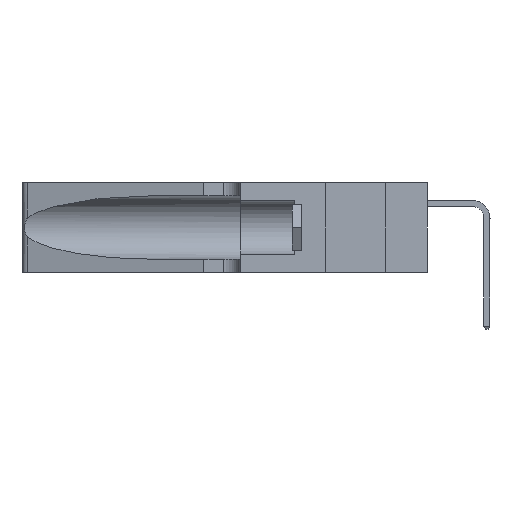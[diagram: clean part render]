
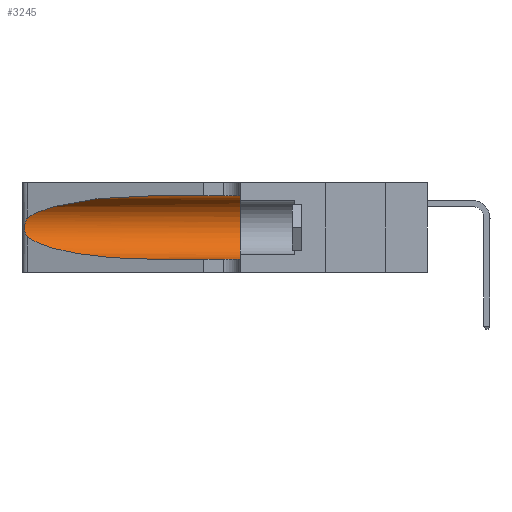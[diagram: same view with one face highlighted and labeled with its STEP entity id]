
A CAD part, left-side view. The second image highlights one B-rep face of the part: STEP entity #3245.
In plain terms, the highlighted cylindrical face has radius 3.308 mm (diameter 6.617 mm), a partial arc.
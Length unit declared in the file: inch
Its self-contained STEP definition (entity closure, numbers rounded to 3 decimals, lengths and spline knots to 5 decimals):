
#115 = EDGE_LOOP ( 'NONE', ( #27801, #45926, #17622, #12856, #36466, #26575 ) ) ;
#1386 = EDGE_CURVE ( 'NONE', #31022, #13780, #26283, .T. ) ;
#2313 = CARTESIAN_POINT ( 'NONE',  ( 0.2373, 1.15595, 0.08982 ) ) ;
#2814 = CARTESIAN_POINT ( 'NONE',  ( 0.26075, 1.23896, 0.19203 ) ) ;
#3019 = CARTESIAN_POINT ( 'NONE',  ( 0.1305, 0.35, 0.185 ) ) ;
#3245 = ADVANCED_FACE ( 'NONE', ( #13210 ), #21720, .F. ) ;
#4918 = EDGE_CURVE ( 'NONE', #27799, #7878, #23805, .T. ) ;
#5717 = CARTESIAN_POINT ( 'NONE',  ( 0.1305, 0.72297, 0.31525 ) ) ;
#6472 = CARTESIAN_POINT ( 'NONE',  ( 0.26017, 1.23833, 0.17102 ) ) ;
#6619 = DIRECTION ( 'NONE',  ( 0., -1., 0. ) ) ;
#6680 = DIRECTION ( 'NONE',  ( 0., 0., 1. ) ) ;
#7878 = VERTEX_POINT ( 'NONE', #38618 ) ;
#8988 = VERTEX_POINT ( 'NONE', #31823 ) ;
#9408 = B_SPLINE_CURVE_WITH_KNOTS ( 'NONE', 3,
 ( #13594, #35331, #42605, #20915, #46248, #24540, #2814, #28203, #6472, #31860, #10105, #35495, #13749, #39148 ),
 .UNSPECIFIED., .F., .F.,
 ( 4, 2, 2, 2, 2, 2, 4 ),
 ( 0., 0.00027, 0.00053, 0.00107, 0.0016, 0.00187, 0.00214 ),
 .UNSPECIFIED. ) ;
#10105 = CARTESIAN_POINT ( 'NONE',  ( 0.25789, 1.23486, 0.15765 ) ) ;
#12316 = CARTESIAN_POINT ( 'NONE',  ( 0.25487, 1.22718, 0.22369 ) ) ;
#12848 = DIRECTION ( 'NONE',  ( 0., -1., 0. ) ) ;
#12856 = ORIENTED_EDGE ( 'NONE', *, *, #4918, .T. ) ;
#13210 = FACE_OUTER_BOUND ( 'NONE', #115, .T. ) ;
#13594 = CARTESIAN_POINT ( 'NONE',  ( 0.25487, 1.22718, 0.22369 ) ) ;
#13749 = CARTESIAN_POINT ( 'NONE',  ( 0.25555, 1.22993, 0.14849 ) ) ;
#13780 = VERTEX_POINT ( 'NONE', #12316 ) ;
#14160 = VECTOR ( 'NONE', #12848, 39.37008 ) ;
#17086 = CARTESIAN_POINT ( 'NONE',  ( 0.1305, 0.72297, 0.05475 ) ) ;
#17622 = ORIENTED_EDGE ( 'NONE', *, *, #38788, .T. ) ;
#20915 = CARTESIAN_POINT ( 'NONE',  ( 0.25787, 1.23484, 0.2124 ) ) ;
#21124 = AXIS2_PLACEMENT_3D ( 'NONE', #28527, #35822, #42935 ) ;
#21473 = VERTEX_POINT ( 'NONE', #31493 ) ;
#21720 = CYLINDRICAL_SURFACE ( 'NONE', #21124, 0.13025 ) ;
#23761 = EDGE_CURVE ( 'NONE', #21473, #7878, #28053, .T. ) ;
#23789 = CARTESIAN_POINT ( 'NONE',  ( 0.2373, 1.15595, 0.28018 ) ) ;
#23805 = LINE ( 'NONE', #38249, #14160 ) ;
#24364 = EDGE_CURVE ( 'NONE', #13780, #8988, #9408, .T. ) ;
#24540 = CARTESIAN_POINT ( 'NONE',  ( 0.26018, 1.23835, 0.19895 ) ) ;
#26219 = LINE ( 'NONE', #28349, #29625 ) ;
#26283 =( BOUNDED_CURVE ( )  B_SPLINE_CURVE ( 3, ( #5717, #27455, #23789, #31104 ),
 .UNSPECIFIED., .F., .F. ) 
 B_SPLINE_CURVE_WITH_KNOTS ( ( 4, 4 ),
 ( 1.5708, 2.84003 ),
 .UNSPECIFIED. ) 
 CURVE ( )  GEOMETRIC_REPRESENTATION_ITEM ( )  RATIONAL_B_SPLINE_CURVE ( ( 1., 0.87, 0.87, 1. ) ) 
 REPRESENTATION_ITEM ( '' )  );
#26575 = ORIENTED_EDGE ( 'NONE', *, *, #35561, .F. ) ;
#27432 = CARTESIAN_POINT ( 'NONE',  ( 0.1305, 0.72297, 0.05475 ) ) ;
#27455 = CARTESIAN_POINT ( 'NONE',  ( 0.18966, 0.96281, 0.31525 ) ) ;
#27799 = VERTEX_POINT ( 'NONE', #27432 ) ;
#27801 = ORIENTED_EDGE ( 'NONE', *, *, #1386, .T. ) ;
#28053 = CIRCLE ( 'NONE', #40078, 0.13025 ) ;
#28203 = CARTESIAN_POINT ( 'NONE',  ( 0.26075, 1.23896, 0.178 ) ) ;
#28349 = CARTESIAN_POINT ( 'NONE',  ( 0.1305, 1.61858, 0.31525 ) ) ;
#28408 = DIRECTION ( 'NONE',  ( 0., 1., 0. ) ) ;
#28527 = CARTESIAN_POINT ( 'NONE',  ( 0.1305, 1.61858, 0.185 ) ) ;
#29625 = VECTOR ( 'NONE', #6619, 39.37008 ) ;
#31022 = VERTEX_POINT ( 'NONE', #42483 ) ;
#31104 = CARTESIAN_POINT ( 'NONE',  ( 0.25487, 1.22718, 0.22369 ) ) ;
#31493 = CARTESIAN_POINT ( 'NONE',  ( 0.1305, 0.35, 0.31525 ) ) ;
#31513 = CARTESIAN_POINT ( 'NONE',  ( 0.25487, 1.22718, 0.14631 ) ) ;
#31823 = CARTESIAN_POINT ( 'NONE',  ( 0.25487, 1.22718, 0.14631 ) ) ;
#31860 = CARTESIAN_POINT ( 'NONE',  ( 0.25856, 1.23593, 0.16098 ) ) ;
#35331 = CARTESIAN_POINT ( 'NONE',  ( 0.25555, 1.22994, 0.2215 ) ) ;
#35495 = CARTESIAN_POINT ( 'NONE',  ( 0.25639, 1.23186, 0.15144 ) ) ;
#35561 = EDGE_CURVE ( 'NONE', #31022, #21473, #26219, .T. ) ;
#35822 = DIRECTION ( 'NONE',  ( 0., -1., 0. ) ) ;
#36466 = ORIENTED_EDGE ( 'NONE', *, *, #23761, .F. ) ;
#38249 = CARTESIAN_POINT ( 'NONE',  ( 0.1305, 1.61858, 0.05475 ) ) ;
#38618 = CARTESIAN_POINT ( 'NONE',  ( 0.1305, 0.35, 0.05475 ) ) ;
#38788 = EDGE_CURVE ( 'NONE', #8988, #27799, #42276, .T. ) ;
#38818 = CARTESIAN_POINT ( 'NONE',  ( 0.18966, 0.96281, 0.05475 ) ) ;
#39148 = CARTESIAN_POINT ( 'NONE',  ( 0.25487, 1.22718, 0.14631 ) ) ;
#40078 = AXIS2_PLACEMENT_3D ( 'NONE', #3019, #28408, #6680 ) ;
#42276 =( BOUNDED_CURVE ( )  B_SPLINE_CURVE ( 3, ( #31513, #2313, #38818, #17086 ),
 .UNSPECIFIED., .F., .T. ) 
 B_SPLINE_CURVE_WITH_KNOTS ( ( 4, 4 ),
 ( 3.44316, 4.71239 ),
 .UNSPECIFIED. ) 
 CURVE ( )  GEOMETRIC_REPRESENTATION_ITEM ( )  RATIONAL_B_SPLINE_CURVE ( ( 1., 0.87, 0.87, 1. ) ) 
 REPRESENTATION_ITEM ( '' )  );
#42483 = CARTESIAN_POINT ( 'NONE',  ( 0.1305, 0.72297, 0.31525 ) ) ;
#42605 = CARTESIAN_POINT ( 'NONE',  ( 0.25639, 1.23184, 0.21858 ) ) ;
#42935 = DIRECTION ( 'NONE',  ( 0., 0., -1. ) ) ;
#45926 = ORIENTED_EDGE ( 'NONE', *, *, #24364, .T. ) ;
#46248 = CARTESIAN_POINT ( 'NONE',  ( 0.25854, 1.2359, 0.20912 ) ) ;
